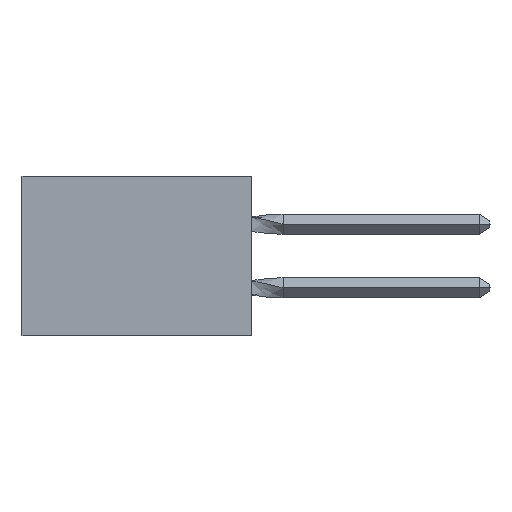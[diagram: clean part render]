
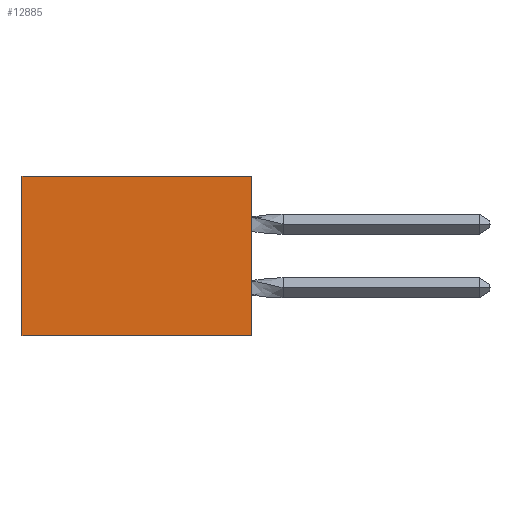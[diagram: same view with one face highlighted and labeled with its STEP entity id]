
A CAD part, left-side view. The second image highlights one B-rep face of the part: STEP entity #12885.
In plain terms, the highlighted planar face has unit normal (-1, 0, 0).
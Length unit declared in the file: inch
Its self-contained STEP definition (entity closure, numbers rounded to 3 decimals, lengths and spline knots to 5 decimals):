
#317 = ORIENTED_EDGE ( 'NONE', *, *, #33511, .F. ) ;
#671 = VERTEX_POINT ( 'NONE', #19992 ) ;
#2967 = VERTEX_POINT ( 'NONE', #23277 ) ;
#5040 = CARTESIAN_POINT ( 'NONE',  ( 0.305, 0., 0. ) ) ;
#5802 = DIRECTION ( 'NONE',  ( 0., 0., -1. ) ) ;
#6238 = AXIS2_PLACEMENT_3D ( 'NONE', #8609, #26970, #5802 ) ;
#6557 = EDGE_CURVE ( 'NONE', #8768, #2967, #29057, .T. ) ;
#7489 = CARTESIAN_POINT ( 'NONE',  ( 0.305, 0., -0.5 ) ) ;
#8609 = CARTESIAN_POINT ( 'NONE',  ( 0.305, 0., -0.5 ) ) ;
#8768 = VERTEX_POINT ( 'NONE', #31528 ) ;
#8872 = ORIENTED_EDGE ( 'NONE', *, *, #18269, .T. ) ;
#10349 = FACE_OUTER_BOUND ( 'NONE', #33588, .T. ) ;
#12885 = ADVANCED_FACE ( 'NONE', ( #10349 ), #18962, .F. ) ;
#13912 = DIRECTION ( 'NONE',  ( 0., 0., -1. ) ) ;
#14874 = VECTOR ( 'NONE', #29489, 39.37008 ) ;
#15576 = LINE ( 'NONE', #7489, #19691 ) ;
#16106 = ORIENTED_EDGE ( 'NONE', *, *, #6557, .T. ) ;
#16600 = CARTESIAN_POINT ( 'NONE',  ( 0.305, 0.72, -0.5 ) ) ;
#17418 = LINE ( 'NONE', #5040, #25674 ) ;
#18269 = EDGE_CURVE ( 'NONE', #671, #8768, #17418, .T. ) ;
#18306 = DIRECTION ( 'NONE',  ( 0., 1., 0. ) ) ;
#18962 = PLANE ( 'NONE',  #6238 ) ;
#19000 = CARTESIAN_POINT ( 'NONE',  ( 0.305, 0., -0.5 ) ) ;
#19691 = VECTOR ( 'NONE', #33934, 39.37008 ) ;
#19992 = CARTESIAN_POINT ( 'NONE',  ( 0.305, 0., 0. ) ) ;
#23174 = VECTOR ( 'NONE', #13912, 39.37008 ) ;
#23277 = CARTESIAN_POINT ( 'NONE',  ( 0.305, 0.72, -0.5 ) ) ;
#25450 = ORIENTED_EDGE ( 'NONE', *, *, #32077, .F. ) ;
#25674 = VECTOR ( 'NONE', #18306, 39.37008 ) ;
#26970 = DIRECTION ( 'NONE',  ( 1., 0., 0. ) ) ;
#27743 = CARTESIAN_POINT ( 'NONE',  ( 0.305, 0., -0.5 ) ) ;
#29057 = LINE ( 'NONE', #16600, #23174 ) ;
#29489 = DIRECTION ( 'NONE',  ( 0., 1., 0. ) ) ;
#30669 = LINE ( 'NONE', #19000, #14874 ) ;
#31528 = CARTESIAN_POINT ( 'NONE',  ( 0.305, 0.72, 0. ) ) ;
#32077 = EDGE_CURVE ( 'NONE', #34467, #2967, #30669, .T. ) ;
#33511 = EDGE_CURVE ( 'NONE', #671, #34467, #15576, .T. ) ;
#33588 = EDGE_LOOP ( 'NONE', ( #16106, #25450, #317, #8872 ) ) ;
#33934 = DIRECTION ( 'NONE',  ( 0., 0., -1. ) ) ;
#34467 = VERTEX_POINT ( 'NONE', #27743 ) ;
